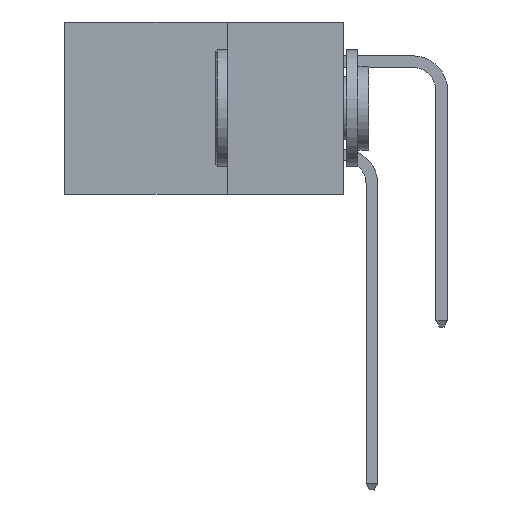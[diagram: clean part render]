
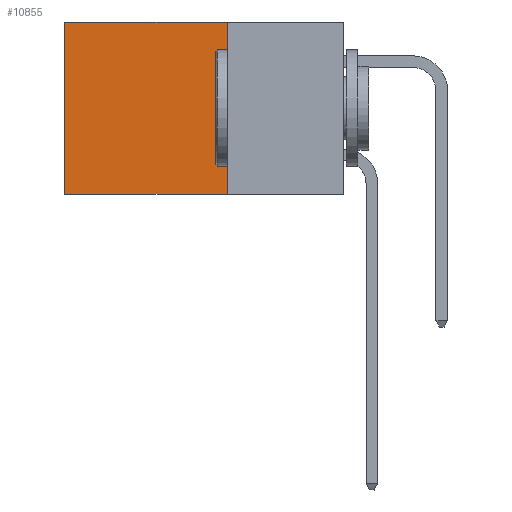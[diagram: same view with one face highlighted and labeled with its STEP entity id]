
A CAD part, left-side view. The second image highlights one B-rep face of the part: STEP entity #10855.
In plain terms, the highlighted planar face has unit normal (-1, 0, 0).
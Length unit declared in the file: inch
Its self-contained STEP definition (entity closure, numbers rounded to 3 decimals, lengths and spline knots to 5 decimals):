
#220 = VECTOR ( 'NONE', #8778, 39.37008 ) ;
#2142 = AXIS2_PLACEMENT_3D ( 'NONE', #14615, #22772, #6598 ) ;
#3786 = ORIENTED_EDGE ( 'NONE', *, *, #27092, .F. ) ;
#3903 = VECTOR ( 'NONE', #24613, 39.37008 ) ;
#4380 = VERTEX_POINT ( 'NONE', #26735 ) ;
#6174 = VECTOR ( 'NONE', #23785, 39.37008 ) ;
#6545 = LINE ( 'NONE', #8389, #3903 ) ;
#6598 = DIRECTION ( 'NONE',  ( 0., 0., -1. ) ) ;
#7069 = VERTEX_POINT ( 'NONE', #29784 ) ;
#7593 = LINE ( 'NONE', #11350, #220 ) ;
#7718 = EDGE_CURVE ( 'NONE', #20422, #7069, #6545, .T. ) ;
#8389 = CARTESIAN_POINT ( 'NONE',  ( 0.298, 0.6, 0. ) ) ;
#8778 = DIRECTION ( 'NONE',  ( 0., 1., 0. ) ) ;
#10855 = ADVANCED_FACE ( 'NONE', ( #11056 ), #20066, .F. ) ;
#11056 = FACE_OUTER_BOUND ( 'NONE', #15711, .T. ) ;
#11350 = CARTESIAN_POINT ( 'NONE',  ( 0.298, 0.25, -0.37 ) ) ;
#11857 = ORIENTED_EDGE ( 'NONE', *, *, #33721, .F. ) ;
#14615 = CARTESIAN_POINT ( 'NONE',  ( 0.298, 0.25, 0. ) ) ;
#14914 = ORIENTED_EDGE ( 'NONE', *, *, #7718, .T. ) ;
#15243 = LINE ( 'NONE', #29050, #28805 ) ;
#15711 = EDGE_LOOP ( 'NONE', ( #14914, #3786, #11857, #20585 ) ) ;
#17534 = CARTESIAN_POINT ( 'NONE',  ( 0.298, 0.6, 0. ) ) ;
#19241 = EDGE_CURVE ( 'NONE', #4380, #20422, #27788, .T. ) ;
#20066 = PLANE ( 'NONE',  #2142 ) ;
#20422 = VERTEX_POINT ( 'NONE', #17534 ) ;
#20585 = ORIENTED_EDGE ( 'NONE', *, *, #19241, .T. ) ;
#21056 = CARTESIAN_POINT ( 'NONE',  ( 0.298, 0.25, 0. ) ) ;
#22772 = DIRECTION ( 'NONE',  ( 1., 0., 0. ) ) ;
#23785 = DIRECTION ( 'NONE',  ( 0., 1., 0. ) ) ;
#24613 = DIRECTION ( 'NONE',  ( 0., 0., -1. ) ) ;
#25531 = VERTEX_POINT ( 'NONE', #34019 ) ;
#26735 = CARTESIAN_POINT ( 'NONE',  ( 0.298, 0.25, 0. ) ) ;
#27092 = EDGE_CURVE ( 'NONE', #25531, #7069, #7593, .T. ) ;
#27788 = LINE ( 'NONE', #21056, #6174 ) ;
#28805 = VECTOR ( 'NONE', #31676, 39.37008 ) ;
#29050 = CARTESIAN_POINT ( 'NONE',  ( 0.298, 0.25, 0. ) ) ;
#29784 = CARTESIAN_POINT ( 'NONE',  ( 0.298, 0.6, -0.37 ) ) ;
#31676 = DIRECTION ( 'NONE',  ( 0., 0., -1. ) ) ;
#33721 = EDGE_CURVE ( 'NONE', #4380, #25531, #15243, .T. ) ;
#34019 = CARTESIAN_POINT ( 'NONE',  ( 0.298, 0.25, -0.37 ) ) ;
